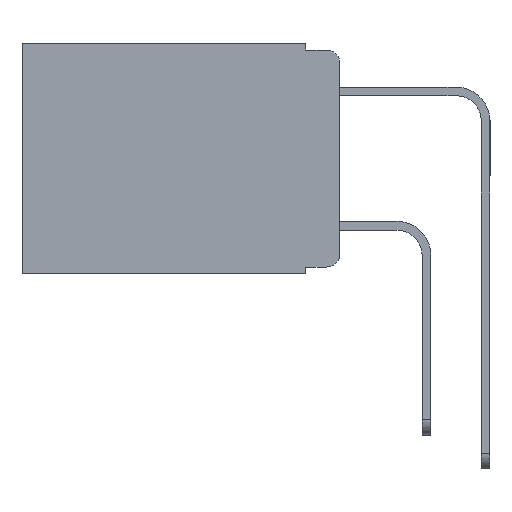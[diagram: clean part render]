
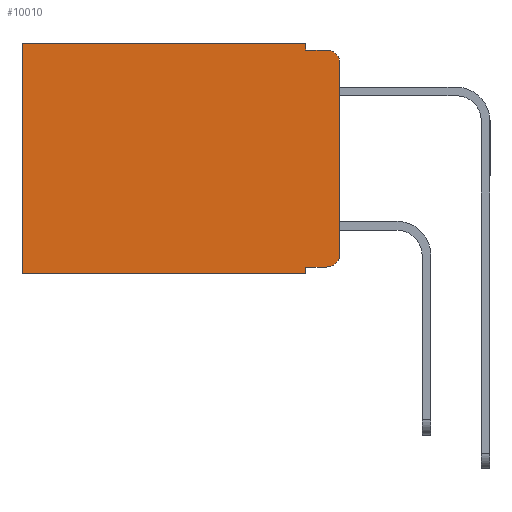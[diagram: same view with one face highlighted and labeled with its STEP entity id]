
A CAD part, left-side view. The second image highlights one B-rep face of the part: STEP entity #10010.
In plain terms, the highlighted planar face has unit normal (-1, 0, 0).
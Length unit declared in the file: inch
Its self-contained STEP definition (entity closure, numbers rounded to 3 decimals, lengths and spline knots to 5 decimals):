
#227 = LINE ( 'NONE', #10334, #16594 ) ;
#1094 = CARTESIAN_POINT ( 'NONE',  ( 0.298, 0.473, 0. ) ) ;
#1380 = EDGE_CURVE ( 'NONE', #3999, #12340, #14329, .T. ) ;
#1882 = DIRECTION ( 'NONE',  ( 0., 0., -1. ) ) ;
#1903 = CARTESIAN_POINT ( 'NONE',  ( 0.298, 0.051, -0.333 ) ) ;
#1963 = VERTEX_POINT ( 'NONE', #6967 ) ;
#2281 = EDGE_CURVE ( 'NONE', #3457, #1963, #7680, .T. ) ;
#2341 = DIRECTION ( 'NONE',  ( 0., 0., -1. ) ) ;
#2597 = VERTEX_POINT ( 'NONE', #8219 ) ;
#2671 = ORIENTED_EDGE ( 'NONE', *, *, #4648, .T. ) ;
#2675 = ORIENTED_EDGE ( 'NONE', *, *, #3179, .F. ) ;
#3021 = EDGE_LOOP ( 'NONE', ( #6817, #3658, #4841, #2675, #2671, #3262, #3610, #7728, #7644, #3926 ) ) ;
#3121 = AXIS2_PLACEMENT_3D ( 'NONE', #5217, #5155, #3972 ) ;
#3179 = EDGE_CURVE ( 'NONE', #2597, #9064, #14293, .T. ) ;
#3262 = ORIENTED_EDGE ( 'NONE', *, *, #2281, .T. ) ;
#3344 = DIRECTION ( 'NONE',  ( 0., 0., -1. ) ) ;
#3457 = VERTEX_POINT ( 'NONE', #1094 ) ;
#3524 = VECTOR ( 'NONE', #2341, 39.37008 ) ;
#3610 = ORIENTED_EDGE ( 'NONE', *, *, #15915, .F. ) ;
#3658 = ORIENTED_EDGE ( 'NONE', *, *, #4379, .T. ) ;
#3911 = LINE ( 'NONE', #1903, #16615 ) ;
#3926 = ORIENTED_EDGE ( 'NONE', *, *, #13107, .T. ) ;
#3972 = DIRECTION ( 'NONE',  ( 0., 0., -1. ) ) ;
#3975 = VECTOR ( 'NONE', #3344, 39.37008 ) ;
#3999 = VERTEX_POINT ( 'NONE', #11617 ) ;
#4379 = EDGE_CURVE ( 'NONE', #3999, #15527, #13468, .T. ) ;
#4648 = EDGE_CURVE ( 'NONE', #2597, #3457, #10276, .T. ) ;
#4841 = ORIENTED_EDGE ( 'NONE', *, *, #4916, .F. ) ;
#4916 = EDGE_CURVE ( 'NONE', #9064, #15527, #227, .T. ) ;
#4953 = LINE ( 'NONE', #7962, #8091 ) ;
#5155 = DIRECTION ( 'NONE',  ( -1., 0., 0. ) ) ;
#5217 = CARTESIAN_POINT ( 'NONE',  ( 0.298, 0.02, -0.03 ) ) ;
#5374 = VERTEX_POINT ( 'NONE', #13299 ) ;
#5430 = LINE ( 'NONE', #8850, #8546 ) ;
#5727 = CARTESIAN_POINT ( 'NONE',  ( 0.298, 0.02, -0.313 ) ) ;
#5813 = CARTESIAN_POINT ( 'NONE',  ( 0.298, 0., 0. ) ) ;
#6526 = AXIS2_PLACEMENT_3D ( 'NONE', #5813, #9801, #1882 ) ;
#6817 = ORIENTED_EDGE ( 'NONE', *, *, #1380, .F. ) ;
#6967 = CARTESIAN_POINT ( 'NONE',  ( 0.298, 0.473, -0.343 ) ) ;
#7063 = DIRECTION ( 'NONE',  ( 0., 0., -1. ) ) ;
#7090 = PLANE ( 'NONE',  #6526 ) ;
#7159 = CIRCLE ( 'NONE', #12394, 0.02 ) ;
#7182 = CARTESIAN_POINT ( 'NONE',  ( 0.298, 0.473, 0. ) ) ;
#7238 = VECTOR ( 'NONE', #8312, 39.37008 ) ;
#7242 = VERTEX_POINT ( 'NONE', #16000 ) ;
#7442 = CARTESIAN_POINT ( 'NONE',  ( 0.298, 0., -0.313 ) ) ;
#7644 = ORIENTED_EDGE ( 'NONE', *, *, #12256, .T. ) ;
#7680 = LINE ( 'NONE', #7182, #7238 ) ;
#7728 = ORIENTED_EDGE ( 'NONE', *, *, #8017, .F. ) ;
#7962 = CARTESIAN_POINT ( 'NONE',  ( 0.298, 0.051, 0. ) ) ;
#8017 = EDGE_CURVE ( 'NONE', #5374, #7242, #4953, .T. ) ;
#8091 = VECTOR ( 'NONE', #11458, 39.37008 ) ;
#8219 = CARTESIAN_POINT ( 'NONE',  ( 0.298, 0.051, 0. ) ) ;
#8312 = DIRECTION ( 'NONE',  ( 0., 0., -1. ) ) ;
#8546 = VECTOR ( 'NONE', #14009, 39.37008 ) ;
#8850 = CARTESIAN_POINT ( 'NONE',  ( 0.298, 0., -0.343 ) ) ;
#9064 = VERTEX_POINT ( 'NONE', #11266 ) ;
#9801 = DIRECTION ( 'NONE',  ( 1., 0., 0. ) ) ;
#10010 = ADVANCED_FACE ( 'NONE', ( #16009 ), #7090, .F. ) ;
#10128 = CARTESIAN_POINT ( 'NONE',  ( 0.298, 0., 0. ) ) ;
#10132 = DIRECTION ( 'NONE',  ( 0., -1., 0. ) ) ;
#10276 = LINE ( 'NONE', #10128, #16409 ) ;
#10334 = CARTESIAN_POINT ( 'NONE',  ( 0.298, 0.051, -0.01 ) ) ;
#11145 = DIRECTION ( 'NONE',  ( 0., -1., 0. ) ) ;
#11266 = CARTESIAN_POINT ( 'NONE',  ( 0.298, 0.051, -0.01 ) ) ;
#11458 = DIRECTION ( 'NONE',  ( 0., 0., -1. ) ) ;
#11617 = CARTESIAN_POINT ( 'NONE',  ( 0.298, 0., -0.03 ) ) ;
#11755 = DIRECTION ( 'NONE',  ( 0., 1., 0. ) ) ;
#12256 = EDGE_CURVE ( 'NONE', #5374, #14986, #3911, .T. ) ;
#12340 = VERTEX_POINT ( 'NONE', #7442 ) ;
#12394 = AXIS2_PLACEMENT_3D ( 'NONE', #5727, #14742, #7063 ) ;
#12997 = CARTESIAN_POINT ( 'NONE',  ( 0.298, 0., 0. ) ) ;
#13107 = EDGE_CURVE ( 'NONE', #14986, #12340, #7159, .T. ) ;
#13299 = CARTESIAN_POINT ( 'NONE',  ( 0.298, 0.051, -0.333 ) ) ;
#13468 = CIRCLE ( 'NONE', #3121, 0.02 ) ;
#14009 = DIRECTION ( 'NONE',  ( 0., 1., 0. ) ) ;
#14084 = CARTESIAN_POINT ( 'NONE',  ( 0.298, 0.051, 0. ) ) ;
#14293 = LINE ( 'NONE', #14084, #3524 ) ;
#14329 = LINE ( 'NONE', #12997, #3975 ) ;
#14588 = CARTESIAN_POINT ( 'NONE',  ( 0.298, 0.02, -0.01 ) ) ;
#14742 = DIRECTION ( 'NONE',  ( -1., 0., 0. ) ) ;
#14941 = CARTESIAN_POINT ( 'NONE',  ( 0.298, 0.02, -0.333 ) ) ;
#14986 = VERTEX_POINT ( 'NONE', #14941 ) ;
#15527 = VERTEX_POINT ( 'NONE', #14588 ) ;
#15915 = EDGE_CURVE ( 'NONE', #7242, #1963, #5430, .T. ) ;
#16000 = CARTESIAN_POINT ( 'NONE',  ( 0.298, 0.051, -0.343 ) ) ;
#16009 = FACE_OUTER_BOUND ( 'NONE', #3021, .T. ) ;
#16409 = VECTOR ( 'NONE', #11755, 39.37008 ) ;
#16594 = VECTOR ( 'NONE', #10132, 39.37008 ) ;
#16615 = VECTOR ( 'NONE', #11145, 39.37008 ) ;
